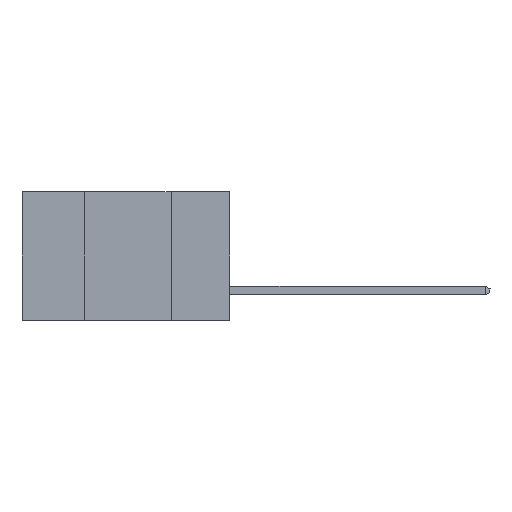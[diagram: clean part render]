
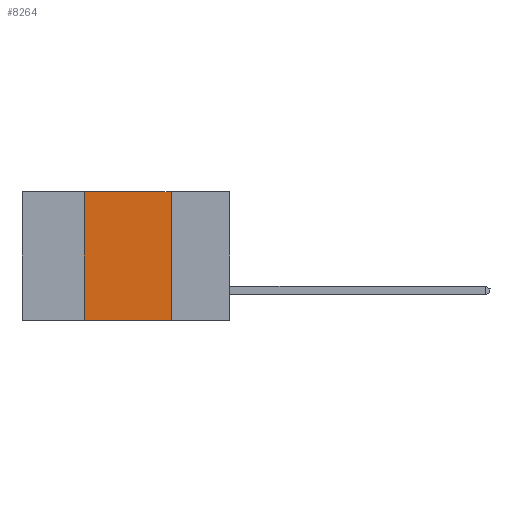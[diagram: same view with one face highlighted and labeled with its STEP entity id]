
A CAD part, left-side view. The second image highlights one B-rep face of the part: STEP entity #8264.
In plain terms, the highlighted planar face has unit normal (-1, 0, 0).
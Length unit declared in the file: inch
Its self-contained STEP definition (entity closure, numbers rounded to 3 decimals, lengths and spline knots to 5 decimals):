
#198 = VERTEX_POINT ( 'NONE', #1883 ) ;
#208 = CARTESIAN_POINT ( 'NONE',  ( 0., 0.6, 0. ) ) ;
#684 = DIRECTION ( 'NONE',  ( 0., 0., 1. ) ) ;
#807 = VERTEX_POINT ( 'NONE', #9691 ) ;
#1539 = CARTESIAN_POINT ( 'NONE',  ( 0., 0.6, -0.37 ) ) ;
#1584 = ORIENTED_EDGE ( 'NONE', *, *, #7283, .F. ) ;
#1883 = CARTESIAN_POINT ( 'NONE',  ( 0., 0.17, 0. ) ) ;
#2028 = FACE_OUTER_BOUND ( 'NONE', #2190, .T. ) ;
#2190 = EDGE_LOOP ( 'NONE', ( #4619, #1584, #6461, #7072 ) ) ;
#2204 = VECTOR ( 'NONE', #7486, 39.37008 ) ;
#2654 = VERTEX_POINT ( 'NONE', #6960 ) ;
#2838 = VECTOR ( 'NONE', #11071, 39.37008 ) ;
#2931 = CARTESIAN_POINT ( 'NONE',  ( 0., 0.42, 0. ) ) ;
#3741 = DIRECTION ( 'NONE',  ( 0., 0., -1. ) ) ;
#4046 = DIRECTION ( 'NONE',  ( 0., -1., 0. ) ) ;
#4590 = AXIS2_PLACEMENT_3D ( 'NONE', #208, #5557, #3741 ) ;
#4619 = ORIENTED_EDGE ( 'NONE', *, *, #5029, .F. ) ;
#4985 = LINE ( 'NONE', #9145, #5839 ) ;
#4986 = CARTESIAN_POINT ( 'NONE',  ( 0., 0.6, 0. ) ) ;
#5029 = EDGE_CURVE ( 'NONE', #198, #807, #10367, .T. ) ;
#5037 = LINE ( 'NONE', #1539, #9480 ) ;
#5557 = DIRECTION ( 'NONE',  ( 1., 0., 0. ) ) ;
#5839 = VECTOR ( 'NONE', #684, 39.37008 ) ;
#6461 = ORIENTED_EDGE ( 'NONE', *, *, #7983, .F. ) ;
#6767 = VERTEX_POINT ( 'NONE', #2931 ) ;
#6960 = CARTESIAN_POINT ( 'NONE',  ( 0., 0.42, -0.37 ) ) ;
#7072 = ORIENTED_EDGE ( 'NONE', *, *, #11017, .T. ) ;
#7283 = EDGE_CURVE ( 'NONE', #6767, #198, #8505, .T. ) ;
#7486 = DIRECTION ( 'NONE',  ( 0., 0., -1. ) ) ;
#7983 = EDGE_CURVE ( 'NONE', #2654, #6767, #4985, .T. ) ;
#8062 = PLANE ( 'NONE',  #4590 ) ;
#8264 = ADVANCED_FACE ( 'NONE', ( #2028 ), #8062, .F. ) ;
#8390 = CARTESIAN_POINT ( 'NONE',  ( 0., 0.17, -0.37 ) ) ;
#8505 = LINE ( 'NONE', #4986, #2838 ) ;
#9145 = CARTESIAN_POINT ( 'NONE',  ( 0., 0.42, -0.37 ) ) ;
#9480 = VECTOR ( 'NONE', #4046, 39.37008 ) ;
#9691 = CARTESIAN_POINT ( 'NONE',  ( 0., 0.17, -0.37 ) ) ;
#10367 = LINE ( 'NONE', #8390, #2204 ) ;
#11017 = EDGE_CURVE ( 'NONE', #2654, #807, #5037, .T. ) ;
#11071 = DIRECTION ( 'NONE',  ( 0., -1., 0. ) ) ;
